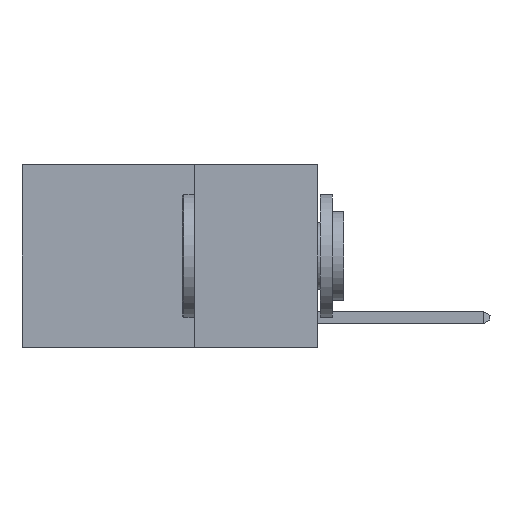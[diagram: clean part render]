
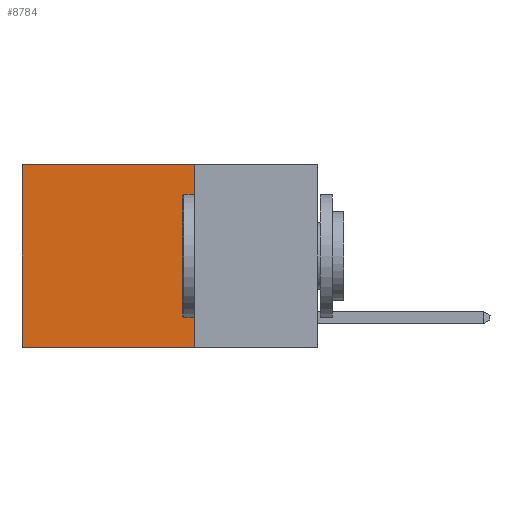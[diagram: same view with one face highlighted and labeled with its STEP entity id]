
A CAD part, left-side view. The second image highlights one B-rep face of the part: STEP entity #8784.
In plain terms, the highlighted planar face has unit normal (-1, 0, 0).
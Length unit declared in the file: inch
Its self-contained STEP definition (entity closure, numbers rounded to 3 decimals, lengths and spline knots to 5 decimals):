
#387 = CARTESIAN_POINT ( 'NONE',  ( 0.2625, 0.25, -0.37 ) ) ;
#587 = VECTOR ( 'NONE', #5092, 39.37008 ) ;
#1523 = ORIENTED_EDGE ( 'NONE', *, *, #1849, .T. ) ;
#1702 = EDGE_CURVE ( 'NONE', #10165, #6799, #4241, .T. ) ;
#1747 = ORIENTED_EDGE ( 'NONE', *, *, #1702, .F. ) ;
#1849 = EDGE_CURVE ( 'NONE', #2646, #8597, #9119, .T. ) ;
#2137 = EDGE_CURVE ( 'NONE', #6799, #8597, #9974, .T. ) ;
#2338 = FACE_OUTER_BOUND ( 'NONE', #4360, .T. ) ;
#2646 = VERTEX_POINT ( 'NONE', #2748 ) ;
#2748 = CARTESIAN_POINT ( 'NONE',  ( 0.2625, 0.6, 0. ) ) ;
#2829 = DIRECTION ( 'NONE',  ( 0., 1., 0. ) ) ;
#3301 = LINE ( 'NONE', #5355, #5725 ) ;
#3600 = CARTESIAN_POINT ( 'NONE',  ( 0.2625, 0.25, 0. ) ) ;
#4241 = LINE ( 'NONE', #8372, #6002 ) ;
#4360 = EDGE_LOOP ( 'NONE', ( #1523, #11028, #1747, #8556 ) ) ;
#4420 = DIRECTION ( 'NONE',  ( 0., 1., 0. ) ) ;
#4582 = CARTESIAN_POINT ( 'NONE',  ( 0.2625, 0.25, 0. ) ) ;
#4937 = CARTESIAN_POINT ( 'NONE',  ( 0.2625, 0.6, 0. ) ) ;
#5092 = DIRECTION ( 'NONE',  ( 0., 0., -1. ) ) ;
#5355 = CARTESIAN_POINT ( 'NONE',  ( 0.2625, 0.25, 0. ) ) ;
#5476 = DIRECTION ( 'NONE',  ( 0., 0., -1. ) ) ;
#5725 = VECTOR ( 'NONE', #4420, 39.37008 ) ;
#6002 = VECTOR ( 'NONE', #8259, 39.37008 ) ;
#6313 = CARTESIAN_POINT ( 'NONE',  ( 0.2625, 0.25, -0.37 ) ) ;
#6799 = VERTEX_POINT ( 'NONE', #387 ) ;
#7111 = CARTESIAN_POINT ( 'NONE',  ( 0.2625, 0.6, -0.37 ) ) ;
#8259 = DIRECTION ( 'NONE',  ( 0., 0., -1. ) ) ;
#8372 = CARTESIAN_POINT ( 'NONE',  ( 0.2625, 0.25, 0. ) ) ;
#8556 = ORIENTED_EDGE ( 'NONE', *, *, #9126, .T. ) ;
#8597 = VERTEX_POINT ( 'NONE', #7111 ) ;
#8784 = ADVANCED_FACE ( 'NONE', ( #2338 ), #8910, .F. ) ;
#8910 = PLANE ( 'NONE',  #9814 ) ;
#9119 = LINE ( 'NONE', #4937, #587 ) ;
#9126 = EDGE_CURVE ( 'NONE', #10165, #2646, #3301, .T. ) ;
#9814 = AXIS2_PLACEMENT_3D ( 'NONE', #4582, #10642, #5476 ) ;
#9845 = VECTOR ( 'NONE', #2829, 39.37008 ) ;
#9974 = LINE ( 'NONE', #6313, #9845 ) ;
#10165 = VERTEX_POINT ( 'NONE', #3600 ) ;
#10642 = DIRECTION ( 'NONE',  ( 1., 0., 0. ) ) ;
#11028 = ORIENTED_EDGE ( 'NONE', *, *, #2137, .F. ) ;
